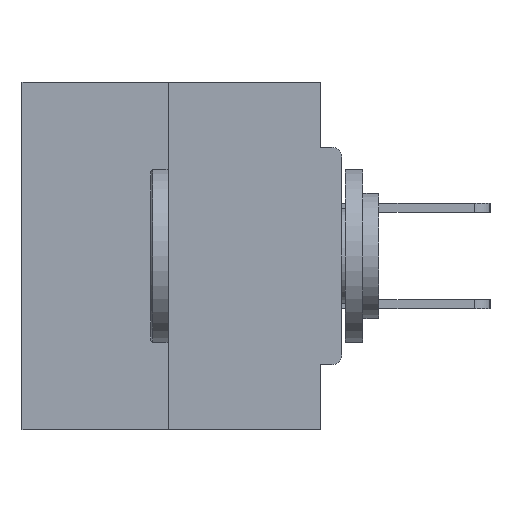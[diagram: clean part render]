
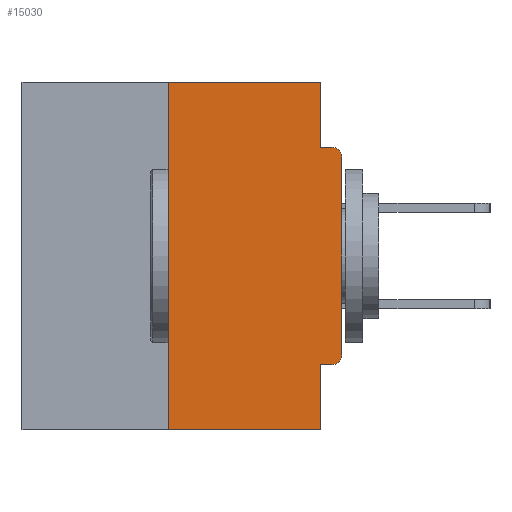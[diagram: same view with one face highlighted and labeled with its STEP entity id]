
A CAD part, left-side view. The second image highlights one B-rep face of the part: STEP entity #15030.
In plain terms, the highlighted planar face has unit normal (-1, 0, 0).
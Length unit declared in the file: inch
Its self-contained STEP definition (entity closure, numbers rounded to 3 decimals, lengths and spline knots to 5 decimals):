
#1090 = LINE ( 'NONE', #30914, #34225 ) ;
#2648 = EDGE_CURVE ( 'NONE', #20660, #22844, #26735, .T. ) ;
#3067 = ORIENTED_EDGE ( 'NONE', *, *, #2648, .T. ) ;
#3707 = CARTESIAN_POINT ( 'NONE',  ( 0., 0., -0.4065 ) ) ;
#4689 = EDGE_CURVE ( 'NONE', #5542, #17982, #39726, .T. ) ;
#5542 = VERTEX_POINT ( 'NONE', #37899 ) ;
#5792 = CARTESIAN_POINT ( 'NONE',  ( 0., 0.015, -0.1085 ) ) ;
#6632 = VECTOR ( 'NONE', #25895, 39.37008 ) ;
#6817 = PLANE ( 'NONE',  #14995 ) ;
#6851 = EDGE_CURVE ( 'NONE', #41552, #8538, #1090, .T. ) ;
#6957 = CIRCLE ( 'NONE', #38247, 0.015 ) ;
#8105 = CARTESIAN_POINT ( 'NONE',  ( 0., 0.031, -0.4065 ) ) ;
#8538 = VERTEX_POINT ( 'NONE', #18160 ) ;
#8595 = EDGE_CURVE ( 'NONE', #17982, #22844, #40964, .T. ) ;
#9124 = ORIENTED_EDGE ( 'NONE', *, *, #14115, .F. ) ;
#9306 = CARTESIAN_POINT ( 'NONE',  ( 0., 0.46, -0.5 ) ) ;
#10264 = EDGE_CURVE ( 'NONE', #5542, #19917, #6957, .T. ) ;
#10736 = VECTOR ( 'NONE', #21177, 39.37008 ) ;
#10979 = VERTEX_POINT ( 'NONE', #41042 ) ;
#12794 = DIRECTION ( 'NONE',  ( 0., 0., -1. ) ) ;
#13257 = AXIS2_PLACEMENT_3D ( 'NONE', #5792, #35837, #28786 ) ;
#13288 = EDGE_CURVE ( 'NONE', #8538, #10979, #24063, .T. ) ;
#14115 = EDGE_CURVE ( 'NONE', #20660, #41552, #37101, .T. ) ;
#14995 = AXIS2_PLACEMENT_3D ( 'NONE', #30393, #20241, #23497 ) ;
#15030 = ADVANCED_FACE ( 'NONE', ( #37562 ), #6817, .F. ) ;
#16269 = VECTOR ( 'NONE', #31521, 39.37008 ) ;
#17068 = CARTESIAN_POINT ( 'NONE',  ( 0., 0.015, -0.0935 ) ) ;
#17294 = DIRECTION ( 'NONE',  ( 0., 1., 0. ) ) ;
#17982 = VERTEX_POINT ( 'NONE', #8105 ) ;
#18013 = CARTESIAN_POINT ( 'NONE',  ( 0., 0.031, 0. ) ) ;
#18160 = CARTESIAN_POINT ( 'NONE',  ( 0., 0.031, 0. ) ) ;
#19011 = CARTESIAN_POINT ( 'NONE',  ( 0., 0.25, -0.5 ) ) ;
#19785 = VERTEX_POINT ( 'NONE', #17068 ) ;
#19917 = VERTEX_POINT ( 'NONE', #38586 ) ;
#20241 = DIRECTION ( 'NONE',  ( 1., 0., 0. ) ) ;
#20660 = VERTEX_POINT ( 'NONE', #19011 ) ;
#21127 = CIRCLE ( 'NONE', #13257, 0.015 ) ;
#21177 = DIRECTION ( 'NONE',  ( 0., 0., 1. ) ) ;
#21820 = VECTOR ( 'NONE', #17294, 39.37008 ) ;
#21923 = ORIENTED_EDGE ( 'NONE', *, *, #8595, .F. ) ;
#22005 = VECTOR ( 'NONE', #22310, 39.37008 ) ;
#22310 = DIRECTION ( 'NONE',  ( 0., -1., 0. ) ) ;
#22660 = CARTESIAN_POINT ( 'NONE',  ( 0., 0., -0.0935 ) ) ;
#22844 = VERTEX_POINT ( 'NONE', #37771 ) ;
#23025 = LINE ( 'NONE', #22660, #6632 ) ;
#23332 = VECTOR ( 'NONE', #40541, 39.37008 ) ;
#23497 = DIRECTION ( 'NONE',  ( 0., 0., -1. ) ) ;
#24063 = LINE ( 'NONE', #18013, #42977 ) ;
#24289 = EDGE_LOOP ( 'NONE', ( #40484, #9124, #3067, #21923, #39400, #34643, #30700, #33005, #28625, #29652 ) ) ;
#25237 = DIRECTION ( 'NONE',  ( 0., 0., -1. ) ) ;
#25895 = DIRECTION ( 'NONE',  ( 0., -1., 0. ) ) ;
#25957 = LINE ( 'NONE', #33646, #23332 ) ;
#26735 = LINE ( 'NONE', #9306, #22005 ) ;
#28625 = ORIENTED_EDGE ( 'NONE', *, *, #29366, .F. ) ;
#28786 = DIRECTION ( 'NONE',  ( 0., 0., -1. ) ) ;
#29366 = EDGE_CURVE ( 'NONE', #10979, #19785, #23025, .T. ) ;
#29652 = ORIENTED_EDGE ( 'NONE', *, *, #13288, .F. ) ;
#30027 = CARTESIAN_POINT ( 'NONE',  ( 0., 0.25, 0. ) ) ;
#30393 = CARTESIAN_POINT ( 'NONE',  ( 0., 0.46, 0. ) ) ;
#30700 = ORIENTED_EDGE ( 'NONE', *, *, #42235, .T. ) ;
#30914 = CARTESIAN_POINT ( 'NONE',  ( 0., 0.46, 0. ) ) ;
#31521 = DIRECTION ( 'NONE',  ( 0., 0., -1. ) ) ;
#33005 = ORIENTED_EDGE ( 'NONE', *, *, #38454, .T. ) ;
#33128 = CARTESIAN_POINT ( 'NONE',  ( 0., 0., -0.1085 ) ) ;
#33646 = CARTESIAN_POINT ( 'NONE',  ( 0., 0., 0. ) ) ;
#33901 = VERTEX_POINT ( 'NONE', #33128 ) ;
#34225 = VECTOR ( 'NONE', #34437, 39.37008 ) ;
#34437 = DIRECTION ( 'NONE',  ( 0., -1., 0. ) ) ;
#34643 = ORIENTED_EDGE ( 'NONE', *, *, #10264, .T. ) ;
#35068 = CARTESIAN_POINT ( 'NONE',  ( 0., 0.031, -0.5 ) ) ;
#35837 = DIRECTION ( 'NONE',  ( -1., 0., 0. ) ) ;
#36341 = DIRECTION ( 'NONE',  ( -1., 0., 0. ) ) ;
#36630 = CARTESIAN_POINT ( 'NONE',  ( 0., 0.015, -0.3915 ) ) ;
#37101 = LINE ( 'NONE', #41160, #10736 ) ;
#37562 = FACE_OUTER_BOUND ( 'NONE', #24289, .T. ) ;
#37771 = CARTESIAN_POINT ( 'NONE',  ( 0., 0.031, -0.5 ) ) ;
#37899 = CARTESIAN_POINT ( 'NONE',  ( 0., 0.015, -0.4065 ) ) ;
#38247 = AXIS2_PLACEMENT_3D ( 'NONE', #36630, #36341, #12794 ) ;
#38454 = EDGE_CURVE ( 'NONE', #33901, #19785, #21127, .T. ) ;
#38586 = CARTESIAN_POINT ( 'NONE',  ( 0., 0., -0.3915 ) ) ;
#39400 = ORIENTED_EDGE ( 'NONE', *, *, #4689, .F. ) ;
#39726 = LINE ( 'NONE', #3707, #21820 ) ;
#40484 = ORIENTED_EDGE ( 'NONE', *, *, #6851, .F. ) ;
#40541 = DIRECTION ( 'NONE',  ( 0., 0., 1. ) ) ;
#40964 = LINE ( 'NONE', #35068, #16269 ) ;
#41042 = CARTESIAN_POINT ( 'NONE',  ( 0., 0.031, -0.0935 ) ) ;
#41160 = CARTESIAN_POINT ( 'NONE',  ( 0., 0.25, 0. ) ) ;
#41552 = VERTEX_POINT ( 'NONE', #30027 ) ;
#42235 = EDGE_CURVE ( 'NONE', #19917, #33901, #25957, .T. ) ;
#42977 = VECTOR ( 'NONE', #25237, 39.37008 ) ;
